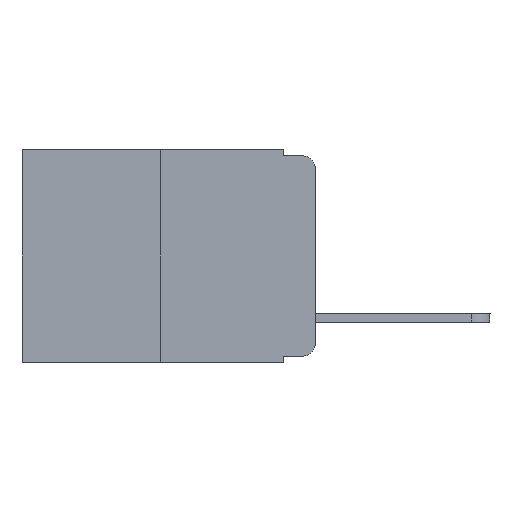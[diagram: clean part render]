
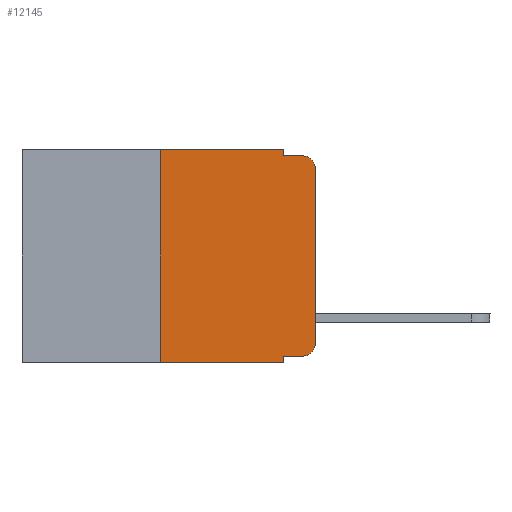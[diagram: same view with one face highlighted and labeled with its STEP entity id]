
A CAD part, left-side view. The second image highlights one B-rep face of the part: STEP entity #12145.
In plain terms, the highlighted planar face has unit normal (-1, 0, 0).
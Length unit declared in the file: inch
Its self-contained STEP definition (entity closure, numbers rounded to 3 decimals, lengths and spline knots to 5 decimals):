
#289 = VERTEX_POINT ( 'NONE', #11599 ) ;
#423 = CARTESIAN_POINT ( 'NONE',  ( 0., 0.02, -0.313 ) ) ;
#434 = DIRECTION ( 'NONE',  ( 0., 0., -1. ) ) ;
#510 = DIRECTION ( 'NONE',  ( 0., 0., -1. ) ) ;
#769 = VERTEX_POINT ( 'NONE', #13669 ) ;
#868 = LINE ( 'NONE', #5996, #13249 ) ;
#883 = DIRECTION ( 'NONE',  ( 0., -1., 0. ) ) ;
#1034 = VECTOR ( 'NONE', #9772, 39.37008 ) ;
#1201 = EDGE_CURVE ( 'NONE', #16527, #289, #15155, .T. ) ;
#1297 = AXIS2_PLACEMENT_3D ( 'NONE', #10765, #8269, #6940 ) ;
#1449 = VECTOR ( 'NONE', #5267, 39.37008 ) ;
#1723 = EDGE_CURVE ( 'NONE', #5567, #5884, #11091, .T. ) ;
#1887 = EDGE_CURVE ( 'NONE', #8730, #5567, #4410, .T. ) ;
#2212 = ORIENTED_EDGE ( 'NONE', *, *, #4543, .T. ) ;
#2506 = AXIS2_PLACEMENT_3D ( 'NONE', #423, #14521, #4110 ) ;
#2684 = CARTESIAN_POINT ( 'NONE',  ( 0., 0.051, 0. ) ) ;
#2975 = VERTEX_POINT ( 'NONE', #7603 ) ;
#3189 = CARTESIAN_POINT ( 'NONE',  ( 0., 0.051, 0. ) ) ;
#3562 = CARTESIAN_POINT ( 'NONE',  ( 0., 0.051, -0.343 ) ) ;
#3685 = EDGE_LOOP ( 'NONE', ( #11122, #2212, #11990, #6541, #13283, #16218, #9447, #15979, #6250, #8616 ) ) ;
#3744 = CARTESIAN_POINT ( 'NONE',  ( 0., 0.051, 0. ) ) ;
#3745 = LINE ( 'NONE', #11197, #5412 ) ;
#3764 = VECTOR ( 'NONE', #510, 39.37008 ) ;
#3841 = EDGE_CURVE ( 'NONE', #12969, #9177, #4626, .T. ) ;
#4041 = PLANE ( 'NONE',  #4699 ) ;
#4110 = DIRECTION ( 'NONE',  ( 0., 0., -1. ) ) ;
#4193 = CARTESIAN_POINT ( 'NONE',  ( 0., 0., 0. ) ) ;
#4410 = CIRCLE ( 'NONE', #2506, 0.02 ) ;
#4543 = EDGE_CURVE ( 'NONE', #5884, #2975, #10662, .T. ) ;
#4626 = LINE ( 'NONE', #4941, #10178 ) ;
#4699 = AXIS2_PLACEMENT_3D ( 'NONE', #11746, #9152, #434 ) ;
#4941 = CARTESIAN_POINT ( 'NONE',  ( 0., 0.25, 0. ) ) ;
#5267 = DIRECTION ( 'NONE',  ( 0., -1., 0. ) ) ;
#5412 = VECTOR ( 'NONE', #8697, 39.37008 ) ;
#5567 = VERTEX_POINT ( 'NONE', #13859 ) ;
#5863 = EDGE_CURVE ( 'NONE', #769, #10150, #11994, .T. ) ;
#5884 = VERTEX_POINT ( 'NONE', #15102 ) ;
#5915 = VECTOR ( 'NONE', #9221, 39.37008 ) ;
#5996 = CARTESIAN_POINT ( 'NONE',  ( 0., 0.473, -0.343 ) ) ;
#6250 = ORIENTED_EDGE ( 'NONE', *, *, #11148, .T. ) ;
#6541 = ORIENTED_EDGE ( 'NONE', *, *, #1201, .F. ) ;
#6922 = FACE_OUTER_BOUND ( 'NONE', #3685, .T. ) ;
#6940 = DIRECTION ( 'NONE',  ( 0., 0., -1. ) ) ;
#7603 = CARTESIAN_POINT ( 'NONE',  ( 0., 0.02, -0.01 ) ) ;
#7831 = DIRECTION ( 'NONE',  ( 0., -1., 0. ) ) ;
#8269 = DIRECTION ( 'NONE',  ( -1., 0., 0. ) ) ;
#8616 = ORIENTED_EDGE ( 'NONE', *, *, #1887, .T. ) ;
#8648 = EDGE_CURVE ( 'NONE', #289, #2975, #3745, .T. ) ;
#8697 = DIRECTION ( 'NONE',  ( 0., -1., 0. ) ) ;
#8730 = VERTEX_POINT ( 'NONE', #11288 ) ;
#9152 = DIRECTION ( 'NONE',  ( 1., 0., 0. ) ) ;
#9177 = VERTEX_POINT ( 'NONE', #16031 ) ;
#9221 = DIRECTION ( 'NONE',  ( 0., 0., 1. ) ) ;
#9447 = ORIENTED_EDGE ( 'NONE', *, *, #11945, .T. ) ;
#9608 = CARTESIAN_POINT ( 'NONE',  ( 0., 0.25, -0.343 ) ) ;
#9772 = DIRECTION ( 'NONE',  ( 0., 0., -1. ) ) ;
#10150 = VERTEX_POINT ( 'NONE', #3562 ) ;
#10178 = VECTOR ( 'NONE', #11455, 39.37008 ) ;
#10234 = EDGE_CURVE ( 'NONE', #9177, #16527, #11097, .T. ) ;
#10662 = CIRCLE ( 'NONE', #1297, 0.02 ) ;
#10765 = CARTESIAN_POINT ( 'NONE',  ( 0., 0.02, -0.03 ) ) ;
#11091 = LINE ( 'NONE', #4193, #5915 ) ;
#11097 = LINE ( 'NONE', #15056, #14551 ) ;
#11122 = ORIENTED_EDGE ( 'NONE', *, *, #1723, .T. ) ;
#11148 = EDGE_CURVE ( 'NONE', #769, #8730, #14226, .T. ) ;
#11197 = CARTESIAN_POINT ( 'NONE',  ( 0., 0.051, -0.01 ) ) ;
#11288 = CARTESIAN_POINT ( 'NONE',  ( 0., 0.02, -0.333 ) ) ;
#11455 = DIRECTION ( 'NONE',  ( 0., 0., 1. ) ) ;
#11599 = CARTESIAN_POINT ( 'NONE',  ( 0., 0.051, -0.01 ) ) ;
#11746 = CARTESIAN_POINT ( 'NONE',  ( 0., 0.473, 0. ) ) ;
#11945 = EDGE_CURVE ( 'NONE', #12969, #10150, #868, .T. ) ;
#11990 = ORIENTED_EDGE ( 'NONE', *, *, #8648, .F. ) ;
#11994 = LINE ( 'NONE', #3189, #3764 ) ;
#12145 = ADVANCED_FACE ( 'NONE', ( #6922 ), #4041, .F. ) ;
#12713 = CARTESIAN_POINT ( 'NONE',  ( 0., 0.051, -0.333 ) ) ;
#12969 = VERTEX_POINT ( 'NONE', #9608 ) ;
#13249 = VECTOR ( 'NONE', #7831, 39.37008 ) ;
#13283 = ORIENTED_EDGE ( 'NONE', *, *, #10234, .F. ) ;
#13669 = CARTESIAN_POINT ( 'NONE',  ( 0., 0.051, -0.333 ) ) ;
#13859 = CARTESIAN_POINT ( 'NONE',  ( 0., 0., -0.313 ) ) ;
#14226 = LINE ( 'NONE', #12713, #1449 ) ;
#14521 = DIRECTION ( 'NONE',  ( -1., 0., 0. ) ) ;
#14551 = VECTOR ( 'NONE', #883, 39.37008 ) ;
#15056 = CARTESIAN_POINT ( 'NONE',  ( 0., 0.473, 0. ) ) ;
#15102 = CARTESIAN_POINT ( 'NONE',  ( 0., 0., -0.03 ) ) ;
#15155 = LINE ( 'NONE', #3744, #1034 ) ;
#15979 = ORIENTED_EDGE ( 'NONE', *, *, #5863, .F. ) ;
#16031 = CARTESIAN_POINT ( 'NONE',  ( 0., 0.25, 0. ) ) ;
#16218 = ORIENTED_EDGE ( 'NONE', *, *, #3841, .F. ) ;
#16527 = VERTEX_POINT ( 'NONE', #2684 ) ;
